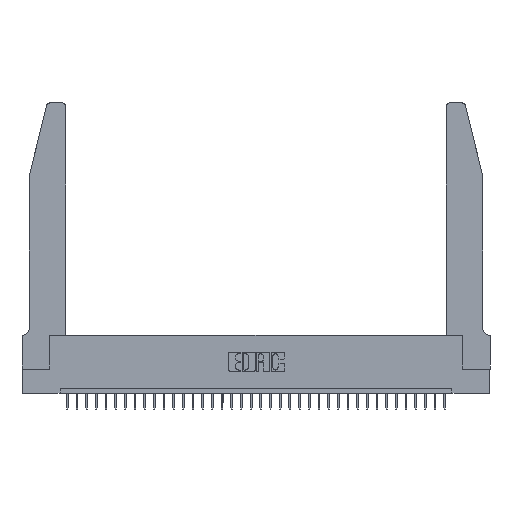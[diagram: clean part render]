
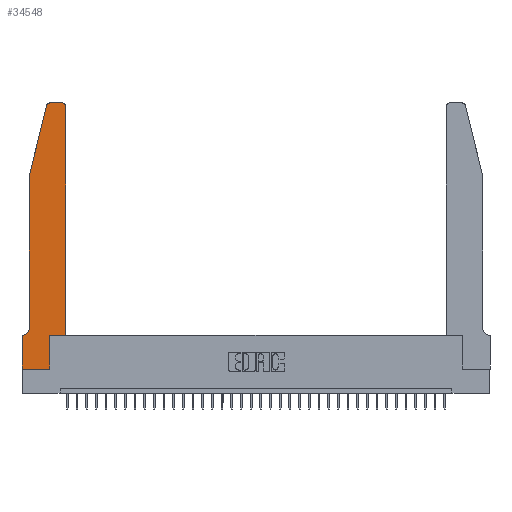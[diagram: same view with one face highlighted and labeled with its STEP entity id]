
A CAD part, top view. The second image highlights one B-rep face of the part: STEP entity #34548.
In plain terms, the highlighted planar face has unit normal (0, 0, 1).
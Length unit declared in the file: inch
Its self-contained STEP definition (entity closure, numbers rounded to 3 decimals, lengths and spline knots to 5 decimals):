
#1469 = DIRECTION ( 'NONE',  ( 0., 0., 1. ) ) ;
#1509 = CARTESIAN_POINT ( 'NONE',  ( 0.0755, 0.42, 0.37 ) ) ;
#2049 = VERTEX_POINT ( 'NONE', #29362 ) ;
#2568 = LINE ( 'NONE', #13126, #16169 ) ;
#2780 = AXIS2_PLACEMENT_3D ( 'NONE', #33874, #20001, #9251 ) ;
#3217 = EDGE_CURVE ( 'NONE', #9406, #27441, #10257, .T. ) ;
#3875 = EDGE_CURVE ( 'NONE', #7829, #4972, #2568, .T. ) ;
#4717 = CIRCLE ( 'NONE', #11998, 0.03 ) ;
#4972 = VERTEX_POINT ( 'NONE', #27741 ) ;
#6261 = CARTESIAN_POINT ( 'NONE',  ( 0.2865, 0.35, 0.37 ) ) ;
#6331 = CARTESIAN_POINT ( 'NONE',  ( 0.0755, 2., 0.37 ) ) ;
#6413 = DIRECTION ( 'NONE',  ( 1., 0., 0. ) ) ;
#6790 = CIRCLE ( 'NONE', #2780, 0.03 ) ;
#7161 = CARTESIAN_POINT ( 'NONE',  ( 0.0055, 0.42, 0.37 ) ) ;
#7663 = VERTEX_POINT ( 'NONE', #22833 ) ;
#7829 = VERTEX_POINT ( 'NONE', #29130 ) ;
#8699 = CIRCLE ( 'NONE', #34885, 0.07 ) ;
#9251 = DIRECTION ( 'NONE',  ( 1., 0., 0. ) ) ;
#9406 = VERTEX_POINT ( 'NONE', #22679 ) ;
#9820 = ORIENTED_EDGE ( 'NONE', *, *, #21581, .T. ) ;
#10257 = LINE ( 'NONE', #6331, #18375 ) ;
#10342 = DIRECTION ( 'NONE',  ( -1., 0., 0. ) ) ;
#10638 = ORIENTED_EDGE ( 'NONE', *, *, #12472, .T. ) ;
#10719 = VERTEX_POINT ( 'NONE', #23909 ) ;
#10847 = VERTEX_POINT ( 'NONE', #20411 ) ;
#10937 = VECTOR ( 'NONE', #12327, 39.37008 ) ;
#11057 = LINE ( 'NONE', #25412, #17988 ) ;
#11354 = VERTEX_POINT ( 'NONE', #20805 ) ;
#11616 = VECTOR ( 'NONE', #30975, 39.37008 ) ;
#11652 = LINE ( 'NONE', #11809, #29577 ) ;
#11809 = CARTESIAN_POINT ( 'NONE',  ( 0.2605, 2.75, 0.37 ) ) ;
#11998 = AXIS2_PLACEMENT_3D ( 'NONE', #12589, #26517, #17963 ) ;
#12327 = DIRECTION ( 'NONE',  ( 1., 0., 0. ) ) ;
#12334 = ORIENTED_EDGE ( 'NONE', *, *, #35211, .T. ) ;
#12472 = EDGE_CURVE ( 'NONE', #19506, #9406, #33185, .T. ) ;
#12589 = CARTESIAN_POINT ( 'NONE',  ( 0.4205, 2.72, 0.37 ) ) ;
#13097 = LINE ( 'NONE', #29630, #19928 ) ;
#13126 = CARTESIAN_POINT ( 'NONE',  ( 0.4505, 0.35, 0.37 ) ) ;
#13138 = CARTESIAN_POINT ( 'NONE',  ( 0.25487, 2.72718, 0.37 ) ) ;
#13354 = DIRECTION ( 'NONE',  ( -0.239, -0.971, 0. ) ) ;
#14038 = VECTOR ( 'NONE', #26883, 39.37008 ) ;
#14522 = EDGE_LOOP ( 'NONE', ( #24612, #22472, #10638, #29216, #23572, #9820, #29387, #12334, #32437, #16636, #27115, #23710 ) ) ;
#14958 = CARTESIAN_POINT ( 'NONE',  ( 0., 0., 0.37 ) ) ;
#16169 = VECTOR ( 'NONE', #23148, 39.37008 ) ;
#16636 = ORIENTED_EDGE ( 'NONE', *, *, #20366, .T. ) ;
#16985 = EDGE_CURVE ( 'NONE', #2049, #10719, #11652, .T. ) ;
#17652 = DIRECTION ( 'NONE',  ( 0., -1., 0. ) ) ;
#17687 = EDGE_CURVE ( 'NONE', #34791, #10847, #21856, .T. ) ;
#17963 = DIRECTION ( 'NONE',  ( 1., 0., 0. ) ) ;
#17988 = VECTOR ( 'NONE', #28255, 39.37008 ) ;
#17995 = DIRECTION ( 'NONE',  ( -1., 0., 0. ) ) ;
#18375 = VECTOR ( 'NONE', #17652, 39.37008 ) ;
#18767 = CARTESIAN_POINT ( 'NONE',  ( 0.2865, 0., 0.37 ) ) ;
#19051 = AXIS2_PLACEMENT_3D ( 'NONE', #25576, #1469, #6413 ) ;
#19506 = VERTEX_POINT ( 'NONE', #13138 ) ;
#19928 = VECTOR ( 'NONE', #10342, 39.37008 ) ;
#20001 = DIRECTION ( 'NONE',  ( 0., 0., 1. ) ) ;
#20366 = EDGE_CURVE ( 'NONE', #10847, #7829, #28559, .T. ) ;
#20411 = CARTESIAN_POINT ( 'NONE',  ( 0.2865, 0.35, 0.37 ) ) ;
#20805 = CARTESIAN_POINT ( 'NONE',  ( 0.0055, 0.35, 0.37 ) ) ;
#20838 = EDGE_CURVE ( 'NONE', #10719, #19506, #6790, .T. ) ;
#21581 = EDGE_CURVE ( 'NONE', #11354, #7663, #13097, .T. ) ;
#21856 = LINE ( 'NONE', #6261, #11616 ) ;
#22472 = ORIENTED_EDGE ( 'NONE', *, *, #20838, .T. ) ;
#22679 = CARTESIAN_POINT ( 'NONE',  ( 0.0755, 2., 0.37 ) ) ;
#22833 = CARTESIAN_POINT ( 'NONE',  ( 0., 0.35, 0.37 ) ) ;
#23148 = DIRECTION ( 'NONE',  ( 0., 1., 0. ) ) ;
#23432 = FACE_OUTER_BOUND ( 'NONE', #14522, .T. ) ;
#23572 = ORIENTED_EDGE ( 'NONE', *, *, #31350, .T. ) ;
#23593 = DIRECTION ( 'NONE',  ( 0., 0., -1. ) ) ;
#23710 = ORIENTED_EDGE ( 'NONE', *, *, #26197, .T. ) ;
#23909 = CARTESIAN_POINT ( 'NONE',  ( 0.284, 2.75, 0.37 ) ) ;
#24612 = ORIENTED_EDGE ( 'NONE', *, *, #16985, .T. ) ;
#25412 = CARTESIAN_POINT ( 'NONE',  ( 0., 0., 0.37 ) ) ;
#25576 = CARTESIAN_POINT ( 'NONE',  ( 0., 0.35, 0.37 ) ) ;
#26032 = VECTOR ( 'NONE', #13354, 39.37008 ) ;
#26197 = EDGE_CURVE ( 'NONE', #4972, #2049, #4717, .T. ) ;
#26517 = DIRECTION ( 'NONE',  ( 0., 0., 1. ) ) ;
#26883 = DIRECTION ( 'NONE',  ( 1., 0., 0. ) ) ;
#26942 = CARTESIAN_POINT ( 'NONE',  ( 0.0755, 2., 0.37 ) ) ;
#27115 = ORIENTED_EDGE ( 'NONE', *, *, #3875, .T. ) ;
#27441 = VERTEX_POINT ( 'NONE', #1509 ) ;
#27741 = CARTESIAN_POINT ( 'NONE',  ( 0.4505, 2.72, 0.37 ) ) ;
#28170 = PLANE ( 'NONE',  #19051 ) ;
#28255 = DIRECTION ( 'NONE',  ( 0., -1., 0. ) ) ;
#28559 = LINE ( 'NONE', #32429, #14038 ) ;
#29130 = CARTESIAN_POINT ( 'NONE',  ( 0.4505, 0.35, 0.37 ) ) ;
#29216 = ORIENTED_EDGE ( 'NONE', *, *, #3217, .T. ) ;
#29362 = CARTESIAN_POINT ( 'NONE',  ( 0.4205, 2.75, 0.37 ) ) ;
#29387 = ORIENTED_EDGE ( 'NONE', *, *, #33472, .T. ) ;
#29577 = VECTOR ( 'NONE', #33561, 39.37008 ) ;
#29630 = CARTESIAN_POINT ( 'NONE',  ( 0.0755, 0.35, 0.37 ) ) ;
#30975 = DIRECTION ( 'NONE',  ( 0., 1., 0. ) ) ;
#31350 = EDGE_CURVE ( 'NONE', #27441, #11354, #8699, .T. ) ;
#32429 = CARTESIAN_POINT ( 'NONE',  ( 0.4505, 0.35, 0.37 ) ) ;
#32437 = ORIENTED_EDGE ( 'NONE', *, *, #17687, .T. ) ;
#32620 = VERTEX_POINT ( 'NONE', #34738 ) ;
#33082 = LINE ( 'NONE', #14958, #10937 ) ;
#33185 = LINE ( 'NONE', #26942, #26032 ) ;
#33472 = EDGE_CURVE ( 'NONE', #7663, #32620, #11057, .T. ) ;
#33561 = DIRECTION ( 'NONE',  ( -1., 0., 0. ) ) ;
#33874 = CARTESIAN_POINT ( 'NONE',  ( 0.284, 2.72, 0.37 ) ) ;
#34548 = ADVANCED_FACE ( 'NONE', ( #23432 ), #28170, .T. ) ;
#34738 = CARTESIAN_POINT ( 'NONE',  ( 0., 0., 0.37 ) ) ;
#34791 = VERTEX_POINT ( 'NONE', #18767 ) ;
#34885 = AXIS2_PLACEMENT_3D ( 'NONE', #7161, #23593, #17995 ) ;
#35211 = EDGE_CURVE ( 'NONE', #32620, #34791, #33082, .T. ) ;
